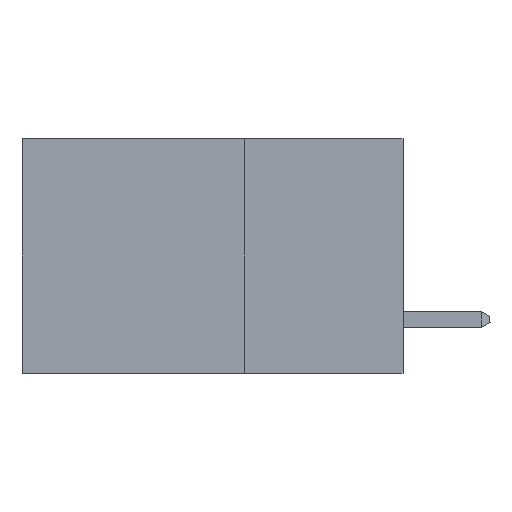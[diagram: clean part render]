
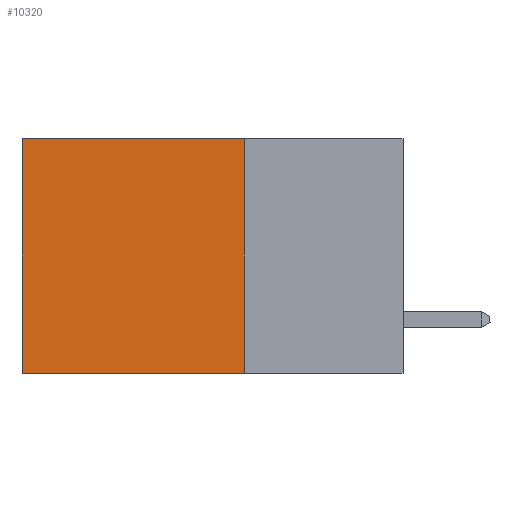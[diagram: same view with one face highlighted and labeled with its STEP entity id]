
A CAD part, left-side view. The second image highlights one B-rep face of the part: STEP entity #10320.
In plain terms, the highlighted planar face has unit normal (-1, 0, 0).
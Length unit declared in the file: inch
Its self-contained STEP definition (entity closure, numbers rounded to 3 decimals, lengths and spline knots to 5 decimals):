
#828 = LINE ( 'NONE', #5391, #4004 ) ;
#992 = CARTESIAN_POINT ( 'NONE',  ( 0.2875, 0.25, -0.37 ) ) ;
#1578 = ORIENTED_EDGE ( 'NONE', *, *, #15076, .F. ) ;
#2049 = EDGE_LOOP ( 'NONE', ( #8224, #17398, #1578, #2460 ) ) ;
#2397 = CARTESIAN_POINT ( 'NONE',  ( 0.2875, 0.6, -0.37 ) ) ;
#2460 = ORIENTED_EDGE ( 'NONE', *, *, #5986, .T. ) ;
#2845 = DIRECTION ( 'NONE',  ( 0., 0., -1. ) ) ;
#3487 = DIRECTION ( 'NONE',  ( 0., 1., 0. ) ) ;
#3793 = VERTEX_POINT ( 'NONE', #2397 ) ;
#3989 = DIRECTION ( 'NONE',  ( 0., 0., -1. ) ) ;
#4004 = VECTOR ( 'NONE', #3989, 39.37008 ) ;
#4052 = DIRECTION ( 'NONE',  ( 1., 0., 0. ) ) ;
#4108 = PLANE ( 'NONE',  #6935 ) ;
#4186 = VECTOR ( 'NONE', #13051, 39.37008 ) ;
#4630 = CARTESIAN_POINT ( 'NONE',  ( 0.2875, 0.25, 0. ) ) ;
#4689 = FACE_OUTER_BOUND ( 'NONE', #2049, .T. ) ;
#5200 = LINE ( 'NONE', #992, #7921 ) ;
#5353 = VECTOR ( 'NONE', #10231, 39.37008 ) ;
#5391 = CARTESIAN_POINT ( 'NONE',  ( 0.2875, 0.25, 0. ) ) ;
#5761 = VERTEX_POINT ( 'NONE', #12296 ) ;
#5986 = EDGE_CURVE ( 'NONE', #16417, #8927, #15712, .T. ) ;
#6935 = AXIS2_PLACEMENT_3D ( 'NONE', #16180, #4052, #2845 ) ;
#7921 = VECTOR ( 'NONE', #3487, 39.37008 ) ;
#8180 = EDGE_CURVE ( 'NONE', #8927, #3793, #16266, .T. ) ;
#8224 = ORIENTED_EDGE ( 'NONE', *, *, #8180, .T. ) ;
#8927 = VERTEX_POINT ( 'NONE', #17166 ) ;
#9835 = CARTESIAN_POINT ( 'NONE',  ( 0.2875, 0.25, 0. ) ) ;
#10231 = DIRECTION ( 'NONE',  ( 0., 0., -1. ) ) ;
#10320 = ADVANCED_FACE ( 'NONE', ( #4689 ), #4108, .F. ) ;
#12296 = CARTESIAN_POINT ( 'NONE',  ( 0.2875, 0.25, -0.37 ) ) ;
#13051 = DIRECTION ( 'NONE',  ( 0., 1., 0. ) ) ;
#14198 = EDGE_CURVE ( 'NONE', #5761, #3793, #5200, .T. ) ;
#15076 = EDGE_CURVE ( 'NONE', #16417, #5761, #828, .T. ) ;
#15712 = LINE ( 'NONE', #4630, #4186 ) ;
#16180 = CARTESIAN_POINT ( 'NONE',  ( 0.2875, 0.25, 0. ) ) ;
#16266 = LINE ( 'NONE', #16935, #5353 ) ;
#16417 = VERTEX_POINT ( 'NONE', #9835 ) ;
#16935 = CARTESIAN_POINT ( 'NONE',  ( 0.2875, 0.6, 0. ) ) ;
#17166 = CARTESIAN_POINT ( 'NONE',  ( 0.2875, 0.6, 0. ) ) ;
#17398 = ORIENTED_EDGE ( 'NONE', *, *, #14198, .F. ) ;
